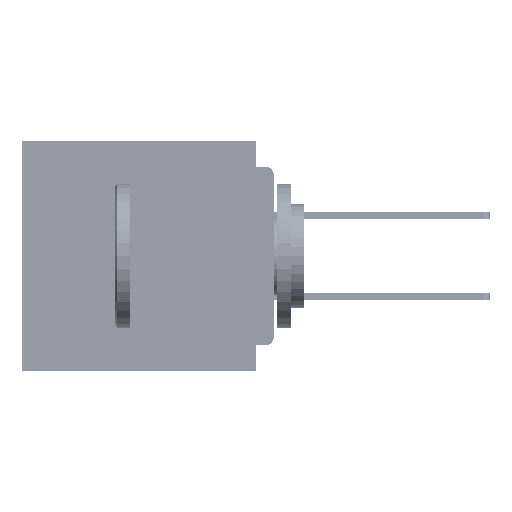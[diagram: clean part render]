
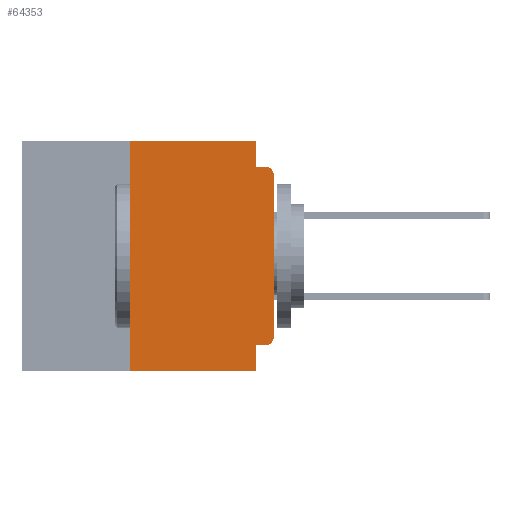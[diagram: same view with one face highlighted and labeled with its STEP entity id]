
A CAD part, left-side view. The second image highlights one B-rep face of the part: STEP entity #64353.
In plain terms, the highlighted planar face has unit normal (-1, 0, 0).
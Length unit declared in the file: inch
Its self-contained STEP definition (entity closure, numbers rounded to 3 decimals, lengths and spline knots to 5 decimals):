
#821 = VERTEX_POINT ( 'NONE', #19732 ) ;
#850 = VERTEX_POINT ( 'NONE', #16521 ) ;
#1244 = DIRECTION ( 'NONE',  ( -1., 0., 0. ) ) ;
#2858 = CARTESIAN_POINT ( 'NONE',  ( 0., 0.25, 0. ) ) ;
#4525 = CARTESIAN_POINT ( 'NONE',  ( 0., 0.031, 0. ) ) ;
#4805 = EDGE_CURVE ( 'NONE', #31870, #850, #64103, .T. ) ;
#6344 = EDGE_CURVE ( 'NONE', #39653, #39656, #15564, .T. ) ;
#6366 = EDGE_CURVE ( 'NONE', #821, #39653, #24912, .T. ) ;
#9014 = VECTOR ( 'NONE', #67630, 39.37008 ) ;
#9977 = DIRECTION ( 'NONE',  ( 0., 0., -1. ) ) ;
#10447 = ORIENTED_EDGE ( 'NONE', *, *, #4805, .F. ) ;
#11443 = CARTESIAN_POINT ( 'NONE',  ( 0., 0., 0. ) ) ;
#11631 = VECTOR ( 'NONE', #69978, 39.37008 ) ;
#11777 = EDGE_CURVE ( 'NONE', #16935, #63764, #49447, .T. ) ;
#11976 = DIRECTION ( 'NONE',  ( 0., 0., 1. ) ) ;
#12096 = ORIENTED_EDGE ( 'NONE', *, *, #45591, .T. ) ;
#13828 = CARTESIAN_POINT ( 'NONE',  ( 0., 0.031, 0. ) ) ;
#14076 = AXIS2_PLACEMENT_3D ( 'NONE', #55057, #22498, #60435 ) ;
#15564 = LINE ( 'NONE', #33462, #52155 ) ;
#16521 = CARTESIAN_POINT ( 'NONE',  ( 0., 0.015, -0.045 ) ) ;
#16935 = VERTEX_POINT ( 'NONE', #44351 ) ;
#17451 = DIRECTION ( 'NONE',  ( 0., -1., 0. ) ) ;
#19732 = CARTESIAN_POINT ( 'NONE',  ( 0., 0.25, -0.4 ) ) ;
#20098 = CARTESIAN_POINT ( 'NONE',  ( 0., 0.031, -0.4 ) ) ;
#21222 = EDGE_LOOP ( 'NONE', ( #36053, #38043, #10447, #38720, #38651, #28638, #12096, #39287, #40654, #58125 ) ) ;
#21299 = CARTESIAN_POINT ( 'NONE',  ( 0., 0., -0.355 ) ) ;
#22498 = DIRECTION ( 'NONE',  ( -1., 0., 0. ) ) ;
#22595 = PLANE ( 'NONE',  #63552 ) ;
#24560 = AXIS2_PLACEMENT_3D ( 'NONE', #33928, #1244, #39397 ) ;
#24912 = LINE ( 'NONE', #61088, #64717 ) ;
#26811 = CIRCLE ( 'NONE', #24560, 0.015 ) ;
#27873 = LINE ( 'NONE', #21299, #11631 ) ;
#28638 = ORIENTED_EDGE ( 'NONE', *, *, #6366, .F. ) ;
#30030 = LINE ( 'NONE', #11443, #42788 ) ;
#31870 = VERTEX_POINT ( 'NONE', #60917 ) ;
#33348 = CARTESIAN_POINT ( 'NONE',  ( 0., 0.437, 0. ) ) ;
#33462 = CARTESIAN_POINT ( 'NONE',  ( 0., 0.437, 0. ) ) ;
#33585 = DIRECTION ( 'NONE',  ( 0., 0., -1. ) ) ;
#33928 = CARTESIAN_POINT ( 'NONE',  ( 0., 0.015, -0.06 ) ) ;
#34170 = VECTOR ( 'NONE', #66221, 39.37008 ) ;
#35348 = CARTESIAN_POINT ( 'NONE',  ( 0., 0.031, -0.4 ) ) ;
#35376 = VECTOR ( 'NONE', #46572, 39.37008 ) ;
#36053 = ORIENTED_EDGE ( 'NONE', *, *, #51191, .T. ) ;
#38015 = LINE ( 'NONE', #35348, #9014 ) ;
#38043 = ORIENTED_EDGE ( 'NONE', *, *, #55209, .T. ) ;
#38651 = ORIENTED_EDGE ( 'NONE', *, *, #6344, .F. ) ;
#38720 = ORIENTED_EDGE ( 'NONE', *, *, #46552, .F. ) ;
#39287 = ORIENTED_EDGE ( 'NONE', *, *, #58217, .F. ) ;
#39387 = CARTESIAN_POINT ( 'NONE',  ( 0., 0.437, -0.4 ) ) ;
#39397 = DIRECTION ( 'NONE',  ( 0., 0., -1. ) ) ;
#39653 = VERTEX_POINT ( 'NONE', #2858 ) ;
#39656 = VERTEX_POINT ( 'NONE', #13828 ) ;
#40654 = ORIENTED_EDGE ( 'NONE', *, *, #57980, .F. ) ;
#41069 = CARTESIAN_POINT ( 'NONE',  ( 0., 0., -0.045 ) ) ;
#42788 = VECTOR ( 'NONE', #49561, 39.37008 ) ;
#43388 = VECTOR ( 'NONE', #9977, 39.37008 ) ;
#44351 = CARTESIAN_POINT ( 'NONE',  ( 0., 0.015, -0.355 ) ) ;
#45091 = LINE ( 'NONE', #4525, #43388 ) ;
#45591 = EDGE_CURVE ( 'NONE', #821, #61014, #62886, .T. ) ;
#46552 = EDGE_CURVE ( 'NONE', #39656, #31870, #45091, .T. ) ;
#46572 = DIRECTION ( 'NONE',  ( 0., -1., 0. ) ) ;
#47372 = CARTESIAN_POINT ( 'NONE',  ( 0., 0., -0.06 ) ) ;
#47511 = FACE_OUTER_BOUND ( 'NONE', #21222, .T. ) ;
#49447 = CIRCLE ( 'NONE', #14076, 0.015 ) ;
#49561 = DIRECTION ( 'NONE',  ( 0., 0., 1. ) ) ;
#51191 = EDGE_CURVE ( 'NONE', #63764, #62206, #30030, .T. ) ;
#51793 = CARTESIAN_POINT ( 'NONE',  ( 0., 0.031, -0.355 ) ) ;
#52155 = VECTOR ( 'NONE', #17451, 39.37008 ) ;
#54742 = VERTEX_POINT ( 'NONE', #51793 ) ;
#55057 = CARTESIAN_POINT ( 'NONE',  ( 0., 0.015, -0.34 ) ) ;
#55209 = EDGE_CURVE ( 'NONE', #62206, #850, #26811, .T. ) ;
#57980 = EDGE_CURVE ( 'NONE', #16935, #54742, #27873, .T. ) ;
#58125 = ORIENTED_EDGE ( 'NONE', *, *, #11777, .T. ) ;
#58217 = EDGE_CURVE ( 'NONE', #54742, #61014, #38015, .T. ) ;
#60435 = DIRECTION ( 'NONE',  ( 0., 0., -1. ) ) ;
#60917 = CARTESIAN_POINT ( 'NONE',  ( 0., 0.031, -0.045 ) ) ;
#61014 = VERTEX_POINT ( 'NONE', #20098 ) ;
#61088 = CARTESIAN_POINT ( 'NONE',  ( 0., 0.25, -0.4 ) ) ;
#62206 = VERTEX_POINT ( 'NONE', #47372 ) ;
#62886 = LINE ( 'NONE', #39387, #34170 ) ;
#63552 = AXIS2_PLACEMENT_3D ( 'NONE', #33348, #65914, #33585 ) ;
#63764 = VERTEX_POINT ( 'NONE', #66210 ) ;
#64103 = LINE ( 'NONE', #41069, #35376 ) ;
#64353 = ADVANCED_FACE ( 'NONE', ( #47511 ), #22595, .F. ) ;
#64717 = VECTOR ( 'NONE', #11976, 39.37008 ) ;
#65914 = DIRECTION ( 'NONE',  ( 1., 0., 0. ) ) ;
#66210 = CARTESIAN_POINT ( 'NONE',  ( 0., 0., -0.34 ) ) ;
#66221 = DIRECTION ( 'NONE',  ( 0., -1., 0. ) ) ;
#67630 = DIRECTION ( 'NONE',  ( 0., 0., -1. ) ) ;
#69978 = DIRECTION ( 'NONE',  ( 0., 1., 0. ) ) ;
